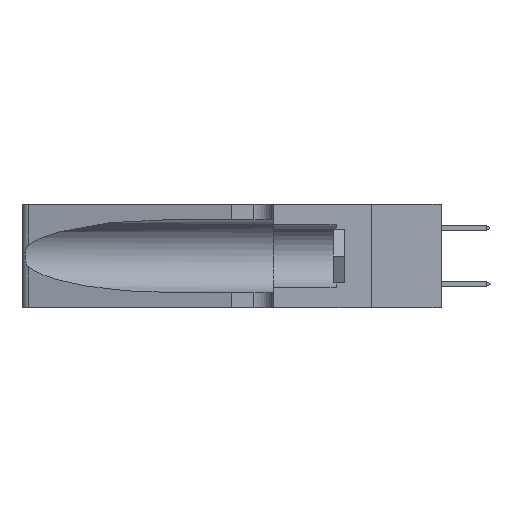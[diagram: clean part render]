
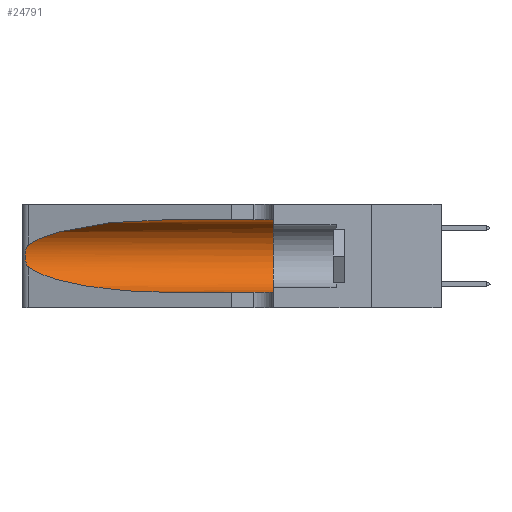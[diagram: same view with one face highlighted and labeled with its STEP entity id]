
A CAD part, left-side view. The second image highlights one B-rep face of the part: STEP entity #24791.
In plain terms, the highlighted cylindrical face has radius 3.308 mm (diameter 6.617 mm), a partial arc.
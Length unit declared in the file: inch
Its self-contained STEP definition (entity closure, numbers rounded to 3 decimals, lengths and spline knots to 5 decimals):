
#227 = CARTESIAN_POINT ( 'NONE',  ( 0.1305, 1.61858, 0.05475 ) ) ;
#716 = DIRECTION ( 'NONE',  ( 0., 1., 0. ) ) ;
#1222 = DIRECTION ( 'NONE',  ( 0., 0., -1. ) ) ;
#2328 = CARTESIAN_POINT ( 'NONE',  ( 0.25854, 1.2359, 0.20912 ) ) ;
#2692 = CARTESIAN_POINT ( 'NONE',  ( 0.1305, 0.72297, 0.31525 ) ) ;
#3223 = DIRECTION ( 'NONE',  ( 0., -1., 0. ) ) ;
#4247 = VERTEX_POINT ( 'NONE', #21408 ) ;
#4519 = CARTESIAN_POINT ( 'NONE',  ( 0.26018, 1.23835, 0.19895 ) ) ;
#4567 = CARTESIAN_POINT ( 'NONE',  ( 0.2373, 1.15595, 0.08982 ) ) ;
#4589 = ORIENTED_EDGE ( 'NONE', *, *, #15599, .T. ) ;
#4701 = CARTESIAN_POINT ( 'NONE',  ( 0.26017, 1.23833, 0.17102 ) ) ;
#5091 = CARTESIAN_POINT ( 'NONE',  ( 0.25789, 1.23486, 0.15765 ) ) ;
#6734 = CARTESIAN_POINT ( 'NONE',  ( 0.1305, 0.72297, 0.05475 ) ) ;
#6858 = EDGE_CURVE ( 'NONE', #25815, #4247, #23939, .T. ) ;
#6962 = CARTESIAN_POINT ( 'NONE',  ( 0.25487, 1.22718, 0.14631 ) ) ;
#7094 = CARTESIAN_POINT ( 'NONE',  ( 0.26075, 1.23896, 0.178 ) ) ;
#7588 = AXIS2_PLACEMENT_3D ( 'NONE', #24731, #3223, #1222 ) ;
#8353 = CARTESIAN_POINT ( 'NONE',  ( 0.1305, 1.61858, 0.31525 ) ) ;
#12814 = EDGE_CURVE ( 'NONE', #17577, #25815, #18058, .T. ) ;
#13012 = AXIS2_PLACEMENT_3D ( 'NONE', #13741, #716, #15945 ) ;
#13159 =( BOUNDED_CURVE ( )  B_SPLINE_CURVE ( 3, ( #6962, #4567, #20050, #17977 ),
 .UNSPECIFIED., .F., .F. ) 
 B_SPLINE_CURVE_WITH_KNOTS ( ( 4, 4 ),
 ( 3.44316, 4.71239 ),
 .UNSPECIFIED. ) 
 CURVE ( )  GEOMETRIC_REPRESENTATION_ITEM ( )  RATIONAL_B_SPLINE_CURVE ( ( 1., 0.87, 0.87, 1. ) ) 
 REPRESENTATION_ITEM ( '' )  );
#13280 = DIRECTION ( 'NONE',  ( 0., -1., 0. ) ) ;
#13318 = CARTESIAN_POINT ( 'NONE',  ( 0.25639, 1.23184, 0.21858 ) ) ;
#13606 = CARTESIAN_POINT ( 'NONE',  ( 0.25856, 1.23593, 0.16098 ) ) ;
#13741 = CARTESIAN_POINT ( 'NONE',  ( 0.1305, 0.35, 0.185 ) ) ;
#13861 = EDGE_CURVE ( 'NONE', #17577, #22250, #22394, .T. ) ;
#15010 = ORIENTED_EDGE ( 'NONE', *, *, #27703, .T. ) ;
#15124 = VECTOR ( 'NONE', #13280, 39.37008 ) ;
#15348 = CARTESIAN_POINT ( 'NONE',  ( 0.25787, 1.23484, 0.2124 ) ) ;
#15530 = CARTESIAN_POINT ( 'NONE',  ( 0.26075, 1.23896, 0.19203 ) ) ;
#15599 = EDGE_CURVE ( 'NONE', #23325, #4247, #16184, .T. ) ;
#15945 = DIRECTION ( 'NONE',  ( 0., 0., 1. ) ) ;
#16184 = LINE ( 'NONE', #227, #15124 ) ;
#16197 = ORIENTED_EDGE ( 'NONE', *, *, #6858, .F. ) ;
#16466 = ORIENTED_EDGE ( 'NONE', *, *, #12814, .F. ) ;
#17024 = B_SPLINE_CURVE_WITH_KNOTS ( 'NONE', 3,
 ( #23936, #28096, #13318, #15348, #2328, #4519, #15530, #7094, #4701, #13606, #5091, #18107, #20276, #19896 ),
 .UNSPECIFIED., .F., .F.,
 ( 4, 2, 2, 2, 2, 2, 4 ),
 ( 0., 0.00027, 0.00053, 0.00107, 0.0016, 0.00187, 0.00214 ),
 .UNSPECIFIED. ) ;
#17374 = VECTOR ( 'NONE', #19025, 39.37008 ) ;
#17577 = VERTEX_POINT ( 'NONE', #18064 ) ;
#17977 = CARTESIAN_POINT ( 'NONE',  ( 0.1305, 0.72297, 0.05475 ) ) ;
#18006 = CARTESIAN_POINT ( 'NONE',  ( 0.18966, 0.96281, 0.31525 ) ) ;
#18058 = LINE ( 'NONE', #8353, #17374 ) ;
#18064 = CARTESIAN_POINT ( 'NONE',  ( 0.1305, 0.72297, 0.31525 ) ) ;
#18107 = CARTESIAN_POINT ( 'NONE',  ( 0.25639, 1.23186, 0.15144 ) ) ;
#18832 = CARTESIAN_POINT ( 'NONE',  ( 0.25487, 1.22718, 0.14631 ) ) ;
#19025 = DIRECTION ( 'NONE',  ( 0., -1., 0. ) ) ;
#19575 = EDGE_LOOP ( 'NONE', ( #24518, #15010, #23604, #4589, #16197, #16466 ) ) ;
#19891 = CARTESIAN_POINT ( 'NONE',  ( 0.1305, 0.35, 0.31525 ) ) ;
#19896 = CARTESIAN_POINT ( 'NONE',  ( 0.25487, 1.22718, 0.14631 ) ) ;
#20050 = CARTESIAN_POINT ( 'NONE',  ( 0.18966, 0.96281, 0.05475 ) ) ;
#20276 = CARTESIAN_POINT ( 'NONE',  ( 0.25555, 1.22993, 0.14849 ) ) ;
#21408 = CARTESIAN_POINT ( 'NONE',  ( 0.1305, 0.35, 0.05475 ) ) ;
#22031 = CYLINDRICAL_SURFACE ( 'NONE', #7588, 0.13025 ) ;
#22250 = VERTEX_POINT ( 'NONE', #27394 ) ;
#22340 = CARTESIAN_POINT ( 'NONE',  ( 0.2373, 1.15595, 0.28018 ) ) ;
#22394 =( BOUNDED_CURVE ( )  B_SPLINE_CURVE ( 3, ( #2692, #18006, #22340, #26360 ),
 .UNSPECIFIED., .F., .F. ) 
 B_SPLINE_CURVE_WITH_KNOTS ( ( 4, 4 ),
 ( 1.5708, 2.84003 ),
 .UNSPECIFIED. ) 
 CURVE ( )  GEOMETRIC_REPRESENTATION_ITEM ( )  RATIONAL_B_SPLINE_CURVE ( ( 1., 0.87, 0.87, 1. ) ) 
 REPRESENTATION_ITEM ( '' )  );
#23325 = VERTEX_POINT ( 'NONE', #6734 ) ;
#23604 = ORIENTED_EDGE ( 'NONE', *, *, #26587, .T. ) ;
#23936 = CARTESIAN_POINT ( 'NONE',  ( 0.25487, 1.22718, 0.22369 ) ) ;
#23939 = CIRCLE ( 'NONE', #13012, 0.13025 ) ;
#24518 = ORIENTED_EDGE ( 'NONE', *, *, #13861, .T. ) ;
#24731 = CARTESIAN_POINT ( 'NONE',  ( 0.1305, 1.61858, 0.185 ) ) ;
#24791 = ADVANCED_FACE ( 'NONE', ( #27770 ), #22031, .F. ) ;
#24930 = VERTEX_POINT ( 'NONE', #18832 ) ;
#25815 = VERTEX_POINT ( 'NONE', #19891 ) ;
#26360 = CARTESIAN_POINT ( 'NONE',  ( 0.25487, 1.22718, 0.22369 ) ) ;
#26587 = EDGE_CURVE ( 'NONE', #24930, #23325, #13159, .T. ) ;
#27394 = CARTESIAN_POINT ( 'NONE',  ( 0.25487, 1.22718, 0.22369 ) ) ;
#27703 = EDGE_CURVE ( 'NONE', #22250, #24930, #17024, .T. ) ;
#27770 = FACE_OUTER_BOUND ( 'NONE', #19575, .T. ) ;
#28096 = CARTESIAN_POINT ( 'NONE',  ( 0.25555, 1.22994, 0.2215 ) ) ;
